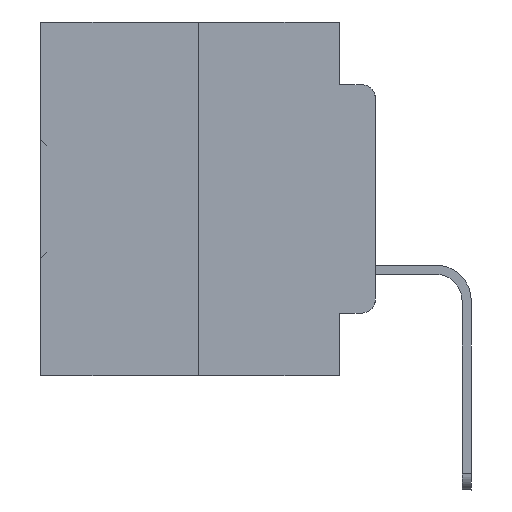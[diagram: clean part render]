
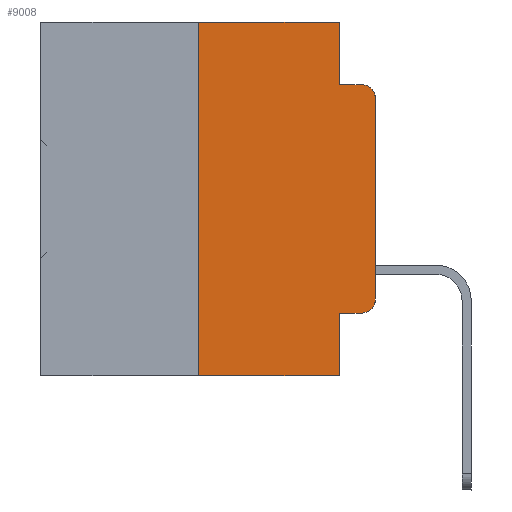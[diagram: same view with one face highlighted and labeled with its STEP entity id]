
A CAD part, left-side view. The second image highlights one B-rep face of the part: STEP entity #9008.
In plain terms, the highlighted planar face has unit normal (-1, 0, 0).
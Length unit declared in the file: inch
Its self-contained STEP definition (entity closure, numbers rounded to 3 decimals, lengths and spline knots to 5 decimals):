
#795 = CARTESIAN_POINT ( 'NONE',  ( 0., 0., 0. ) ) ;
#1474 = CARTESIAN_POINT ( 'NONE',  ( 0., 0.25, -0.5 ) ) ;
#1598 = LINE ( 'NONE', #6333, #29359 ) ;
#1691 = CARTESIAN_POINT ( 'NONE',  ( 0., 0.051, -0.4115 ) ) ;
#2029 = ORIENTED_EDGE ( 'NONE', *, *, #34036, .T. ) ;
#2380 = CIRCLE ( 'NONE', #8150, 0.02 ) ;
#3364 = LINE ( 'NONE', #34651, #25120 ) ;
#4179 = EDGE_CURVE ( 'NONE', #25097, #31637, #26551, .T. ) ;
#4423 = PLANE ( 'NONE',  #25606 ) ;
#4541 = EDGE_CURVE ( 'NONE', #20338, #14332, #11114, .T. ) ;
#4709 = DIRECTION ( 'NONE',  ( 0., -1., 0. ) ) ;
#4782 = VECTOR ( 'NONE', #7513, 39.37008 ) ;
#5404 = CARTESIAN_POINT ( 'NONE',  ( 0., 0.051, -0.5 ) ) ;
#6333 = CARTESIAN_POINT ( 'NONE',  ( 0., 0.051, 0. ) ) ;
#6599 = FACE_OUTER_BOUND ( 'NONE', #25599, .T. ) ;
#6704 = DIRECTION ( 'NONE',  ( 0., 0., -1. ) ) ;
#7513 = DIRECTION ( 'NONE',  ( 0., 0., 1. ) ) ;
#8150 = AXIS2_PLACEMENT_3D ( 'NONE', #9295, #12462, #17481 ) ;
#8207 = CARTESIAN_POINT ( 'NONE',  ( 0., 0.02, -0.1085 ) ) ;
#9008 = ADVANCED_FACE ( 'NONE', ( #6599 ), #4423, .F. ) ;
#9038 = VECTOR ( 'NONE', #9409, 39.37008 ) ;
#9290 = LINE ( 'NONE', #9747, #24600 ) ;
#9295 = CARTESIAN_POINT ( 'NONE',  ( 0., 0.02, -0.3915 ) ) ;
#9409 = DIRECTION ( 'NONE',  ( 0., 0., 1. ) ) ;
#9747 = CARTESIAN_POINT ( 'NONE',  ( 0., 0.051, 0. ) ) ;
#9921 = DIRECTION ( 'NONE',  ( 0., 0., -1. ) ) ;
#10023 = CARTESIAN_POINT ( 'NONE',  ( 0., 0.473, 0. ) ) ;
#10326 = ORIENTED_EDGE ( 'NONE', *, *, #4541, .T. ) ;
#10705 = CARTESIAN_POINT ( 'NONE',  ( 0., 0.25, 0. ) ) ;
#11114 = LINE ( 'NONE', #795, #9038 ) ;
#11208 = DIRECTION ( 'NONE',  ( 0., -1., 0. ) ) ;
#11228 = VECTOR ( 'NONE', #11208, 39.37008 ) ;
#11550 = LINE ( 'NONE', #1691, #33319 ) ;
#11553 = VERTEX_POINT ( 'NONE', #5404 ) ;
#11957 = ORIENTED_EDGE ( 'NONE', *, *, #18668, .F. ) ;
#12462 = DIRECTION ( 'NONE',  ( -1., 0., 0. ) ) ;
#12966 = CARTESIAN_POINT ( 'NONE',  ( 0., 0.25, 0. ) ) ;
#13274 = DIRECTION ( 'NONE',  ( 0., 0., -1. ) ) ;
#13677 = AXIS2_PLACEMENT_3D ( 'NONE', #8207, #35262, #22004 ) ;
#13921 = VERTEX_POINT ( 'NONE', #20615 ) ;
#14332 = VERTEX_POINT ( 'NONE', #25092 ) ;
#14405 = CARTESIAN_POINT ( 'NONE',  ( 0., 0.473, -0.5 ) ) ;
#15220 = VERTEX_POINT ( 'NONE', #35334 ) ;
#15427 = ORIENTED_EDGE ( 'NONE', *, *, #27899, .T. ) ;
#15665 = ORIENTED_EDGE ( 'NONE', *, *, #4179, .F. ) ;
#15687 = EDGE_CURVE ( 'NONE', #25920, #21345, #11550, .T. ) ;
#16705 = CARTESIAN_POINT ( 'NONE',  ( 0., 0.051, 0. ) ) ;
#16924 = CIRCLE ( 'NONE', #13677, 0.02 ) ;
#17165 = VERTEX_POINT ( 'NONE', #16705 ) ;
#17481 = DIRECTION ( 'NONE',  ( 0., 0., -1. ) ) ;
#17698 = EDGE_CURVE ( 'NONE', #31637, #17165, #3364, .T. ) ;
#18668 = EDGE_CURVE ( 'NONE', #25920, #11553, #1598, .T. ) ;
#19514 = EDGE_CURVE ( 'NONE', #17165, #15220, #9290, .T. ) ;
#19586 = ORIENTED_EDGE ( 'NONE', *, *, #19514, .F. ) ;
#19607 = CARTESIAN_POINT ( 'NONE',  ( 0., 0., -0.3915 ) ) ;
#20338 = VERTEX_POINT ( 'NONE', #19607 ) ;
#20615 = CARTESIAN_POINT ( 'NONE',  ( 0., 0.02, -0.0885 ) ) ;
#21345 = VERTEX_POINT ( 'NONE', #22629 ) ;
#22004 = DIRECTION ( 'NONE',  ( 0., 0., -1. ) ) ;
#22629 = CARTESIAN_POINT ( 'NONE',  ( 0., 0.02, -0.4115 ) ) ;
#22739 = CARTESIAN_POINT ( 'NONE',  ( 0., 0.051, -0.0885 ) ) ;
#23023 = LINE ( 'NONE', #22739, #34999 ) ;
#23475 = DIRECTION ( 'NONE',  ( 1., 0., 0. ) ) ;
#24600 = VECTOR ( 'NONE', #13274, 39.37008 ) ;
#25092 = CARTESIAN_POINT ( 'NONE',  ( 0., 0., -0.1085 ) ) ;
#25097 = VERTEX_POINT ( 'NONE', #1474 ) ;
#25120 = VECTOR ( 'NONE', #4709, 39.37008 ) ;
#25599 = EDGE_LOOP ( 'NONE', ( #10326, #15427, #28239, #19586, #27278, #15665, #2029, #11957, #30881, #30860 ) ) ;
#25606 = AXIS2_PLACEMENT_3D ( 'NONE', #10023, #23475, #9921 ) ;
#25920 = VERTEX_POINT ( 'NONE', #30034 ) ;
#26551 = LINE ( 'NONE', #12966, #4782 ) ;
#27278 = ORIENTED_EDGE ( 'NONE', *, *, #17698, .F. ) ;
#27899 = EDGE_CURVE ( 'NONE', #14332, #13921, #16924, .T. ) ;
#28239 = ORIENTED_EDGE ( 'NONE', *, *, #29945, .F. ) ;
#29359 = VECTOR ( 'NONE', #6704, 39.37008 ) ;
#29945 = EDGE_CURVE ( 'NONE', #15220, #13921, #23023, .T. ) ;
#30034 = CARTESIAN_POINT ( 'NONE',  ( 0., 0.051, -0.4115 ) ) ;
#30860 = ORIENTED_EDGE ( 'NONE', *, *, #32885, .T. ) ;
#30881 = ORIENTED_EDGE ( 'NONE', *, *, #15687, .T. ) ;
#31339 = LINE ( 'NONE', #14405, #11228 ) ;
#31637 = VERTEX_POINT ( 'NONE', #10705 ) ;
#32885 = EDGE_CURVE ( 'NONE', #21345, #20338, #2380, .T. ) ;
#33319 = VECTOR ( 'NONE', #34271, 39.37008 ) ;
#33881 = DIRECTION ( 'NONE',  ( 0., -1., 0. ) ) ;
#34036 = EDGE_CURVE ( 'NONE', #25097, #11553, #31339, .T. ) ;
#34271 = DIRECTION ( 'NONE',  ( 0., -1., 0. ) ) ;
#34651 = CARTESIAN_POINT ( 'NONE',  ( 0., 0.473, 0. ) ) ;
#34999 = VECTOR ( 'NONE', #33881, 39.37008 ) ;
#35262 = DIRECTION ( 'NONE',  ( -1., 0., 0. ) ) ;
#35334 = CARTESIAN_POINT ( 'NONE',  ( 0., 0.051, -0.0885 ) ) ;
